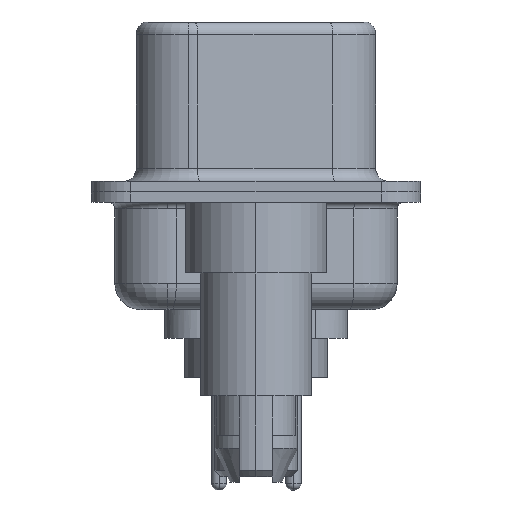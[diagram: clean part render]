
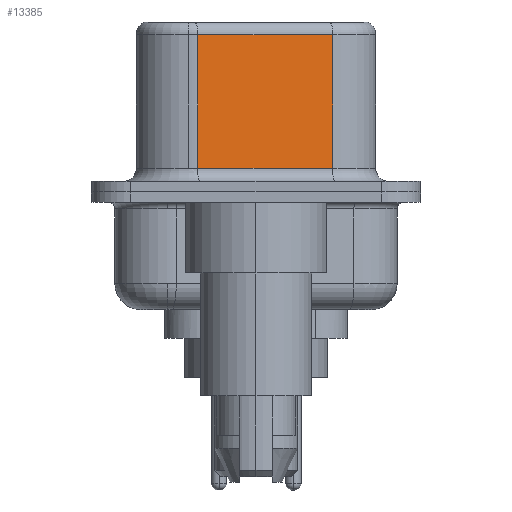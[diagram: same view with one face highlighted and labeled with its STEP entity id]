
A CAD part, left-side view. The second image highlights one B-rep face of the part: STEP entity #13385.
In plain terms, the highlighted planar face has unit normal (-0.985, -0.174, 0).
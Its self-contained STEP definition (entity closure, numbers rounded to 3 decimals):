
#550 = ORIENTED_EDGE ( 'NONE', *, *, #17219, .T. ) ;
#746 = PLANE ( 'NONE',  #3591 ) ;
#1527 = ORIENTED_EDGE ( 'NONE', *, *, #17561, .F. ) ;
#2035 = VERTEX_POINT ( 'NONE', #18833 ) ;
#2322 = LINE ( 'NONE', #21648, #16630 ) ;
#2423 = VECTOR ( 'NONE', #13872, 1000. ) ;
#2435 = VERTEX_POINT ( 'NONE', #10159 ) ;
#2733 = LINE ( 'NONE', #19109, #7438 ) ;
#3591 = AXIS2_PLACEMENT_3D ( 'NONE', #13315, #15114, #4368 ) ;
#4368 = DIRECTION ( 'NONE',  ( -0.174, 0.985, 0. ) ) ;
#5417 = DIRECTION ( 'NONE',  ( 0.174, -0.985, 0. ) ) ;
#7438 = VECTOR ( 'NONE', #8287, 1000. ) ;
#8270 = LINE ( 'NONE', #11962, #2423 ) ;
#8287 = DIRECTION ( 'NONE',  ( 0., 0., -1. ) ) ;
#8716 = CARTESIAN_POINT ( 'NONE',  ( 4.585, -2.927, 6.02 ) ) ;
#10159 = CARTESIAN_POINT ( 'NONE',  ( 3.675, 2.233, 0.9 ) ) ;
#10417 = LINE ( 'NONE', #11645, #14663 ) ;
#11645 = CARTESIAN_POINT ( 'NONE',  ( 4.585, -2.927, 6.52 ) ) ;
#11962 = CARTESIAN_POINT ( 'NONE',  ( 4.585, -2.927, 6.02 ) ) ;
#13315 = CARTESIAN_POINT ( 'NONE',  ( 4.585, -2.927, 6.52 ) ) ;
#13385 = ADVANCED_FACE ( 'NONE', ( #17955 ), #746, .F. ) ;
#13747 = VERTEX_POINT ( 'NONE', #8716 ) ;
#13872 = DIRECTION ( 'NONE',  ( -0.174, 0.985, 0. ) ) ;
#14129 = VERTEX_POINT ( 'NONE', #20561 ) ;
#14663 = VECTOR ( 'NONE', #15273, 1000. ) ;
#15114 = DIRECTION ( 'NONE',  ( 0.985, 0.174, 0. ) ) ;
#15273 = DIRECTION ( 'NONE',  ( 0., 0., -1. ) ) ;
#16187 = ORIENTED_EDGE ( 'NONE', *, *, #21273, .T. ) ;
#16630 = VECTOR ( 'NONE', #5417, 1000. ) ;
#17219 = EDGE_CURVE ( 'NONE', #2435, #2035, #2322, .T. ) ;
#17561 = EDGE_CURVE ( 'NONE', #13747, #2035, #10417, .T. ) ;
#17929 = EDGE_LOOP ( 'NONE', ( #1527, #22601, #16187, #550 ) ) ;
#17955 = FACE_OUTER_BOUND ( 'NONE', #17929, .T. ) ;
#18833 = CARTESIAN_POINT ( 'NONE',  ( 4.585, -2.927, 0.9 ) ) ;
#19109 = CARTESIAN_POINT ( 'NONE',  ( 3.675, 2.233, 6.52 ) ) ;
#20561 = CARTESIAN_POINT ( 'NONE',  ( 3.675, 2.233, 6.02 ) ) ;
#21273 = EDGE_CURVE ( 'NONE', #14129, #2435, #2733, .T. ) ;
#21648 = CARTESIAN_POINT ( 'NONE',  ( 4.585, -2.927, 0.9 ) ) ;
#22096 = EDGE_CURVE ( 'NONE', #13747, #14129, #8270, .T. ) ;
#22601 = ORIENTED_EDGE ( 'NONE', *, *, #22096, .T. ) ;
